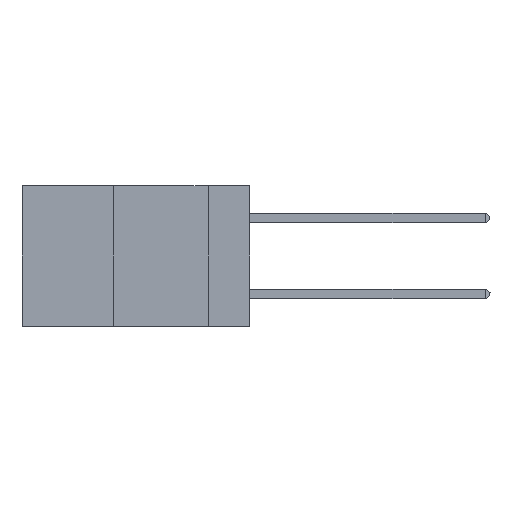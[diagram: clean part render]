
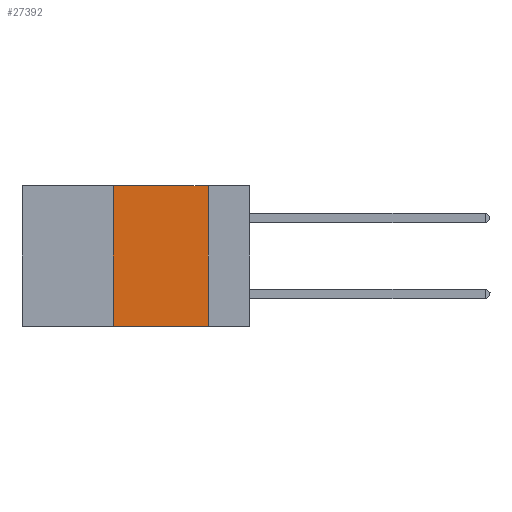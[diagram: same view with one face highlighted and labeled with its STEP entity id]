
A CAD part, left-side view. The second image highlights one B-rep face of the part: STEP entity #27392.
In plain terms, the highlighted planar face has unit normal (-1, 0, 0).
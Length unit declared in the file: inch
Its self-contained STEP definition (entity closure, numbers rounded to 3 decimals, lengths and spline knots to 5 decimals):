
#3140 = EDGE_CURVE ( 'NONE', #16696, #32283, #4851, .T. ) ;
#3346 = EDGE_CURVE ( 'NONE', #31116, #28185, #27574, .T. ) ;
#4851 = LINE ( 'NONE', #36837, #28052 ) ;
#5585 = CARTESIAN_POINT ( 'NONE',  ( 0., 0.11, -0.37 ) ) ;
#5715 = CARTESIAN_POINT ( 'NONE',  ( 0., 0.6, 0. ) ) ;
#7653 = CARTESIAN_POINT ( 'NONE',  ( 0., 0.36, -0.37 ) ) ;
#7809 = ORIENTED_EDGE ( 'NONE', *, *, #3140, .T. ) ;
#11568 = DIRECTION ( 'NONE',  ( 0., 0., -1. ) ) ;
#13800 = ORIENTED_EDGE ( 'NONE', *, *, #14814, .F. ) ;
#14353 = PLANE ( 'NONE',  #36027 ) ;
#14814 = EDGE_CURVE ( 'NONE', #16696, #31116, #15111, .T. ) ;
#15111 = LINE ( 'NONE', #17353, #37234 ) ;
#16679 = DIRECTION ( 'NONE',  ( 0., -1., 0. ) ) ;
#16696 = VERTEX_POINT ( 'NONE', #7653 ) ;
#17353 = CARTESIAN_POINT ( 'NONE',  ( 0., 0.36, 0. ) ) ;
#19428 = DIRECTION ( 'NONE',  ( 0., 0., -1. ) ) ;
#19868 = VECTOR ( 'NONE', #21864, 39.37008 ) ;
#21591 = FACE_OUTER_BOUND ( 'NONE', #36561, .T. ) ;
#21864 = DIRECTION ( 'NONE',  ( 0., -1., 0. ) ) ;
#22891 = ORIENTED_EDGE ( 'NONE', *, *, #24570, .F. ) ;
#23836 = CARTESIAN_POINT ( 'NONE',  ( 0., 0.36, 0. ) ) ;
#24570 = EDGE_CURVE ( 'NONE', #28185, #32283, #25920, .T. ) ;
#25002 = VECTOR ( 'NONE', #19428, 39.37008 ) ;
#25920 = LINE ( 'NONE', #33832, #25002 ) ;
#27392 = ADVANCED_FACE ( 'NONE', ( #21591 ), #14353, .F. ) ;
#27574 = LINE ( 'NONE', #33390, #19868 ) ;
#28052 = VECTOR ( 'NONE', #16679, 39.37008 ) ;
#28185 = VERTEX_POINT ( 'NONE', #36233 ) ;
#28975 = DIRECTION ( 'NONE',  ( 1., 0., 0. ) ) ;
#31116 = VERTEX_POINT ( 'NONE', #23836 ) ;
#32283 = VERTEX_POINT ( 'NONE', #5585 ) ;
#33390 = CARTESIAN_POINT ( 'NONE',  ( 0., 0.6, 0. ) ) ;
#33832 = CARTESIAN_POINT ( 'NONE',  ( 0., 0.11, 0. ) ) ;
#34643 = DIRECTION ( 'NONE',  ( 0., 0., 1. ) ) ;
#36027 = AXIS2_PLACEMENT_3D ( 'NONE', #5715, #28975, #11568 ) ;
#36233 = CARTESIAN_POINT ( 'NONE',  ( 0., 0.11, 0. ) ) ;
#36506 = ORIENTED_EDGE ( 'NONE', *, *, #3346, .F. ) ;
#36561 = EDGE_LOOP ( 'NONE', ( #22891, #36506, #13800, #7809 ) ) ;
#36837 = CARTESIAN_POINT ( 'NONE',  ( 0., 0.6, -0.37 ) ) ;
#37234 = VECTOR ( 'NONE', #34643, 39.37008 ) ;
